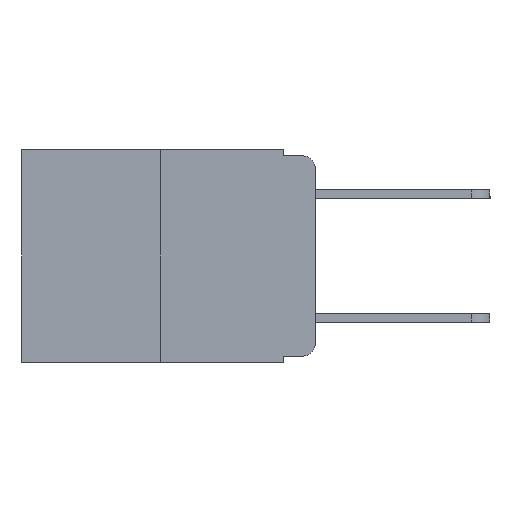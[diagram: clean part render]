
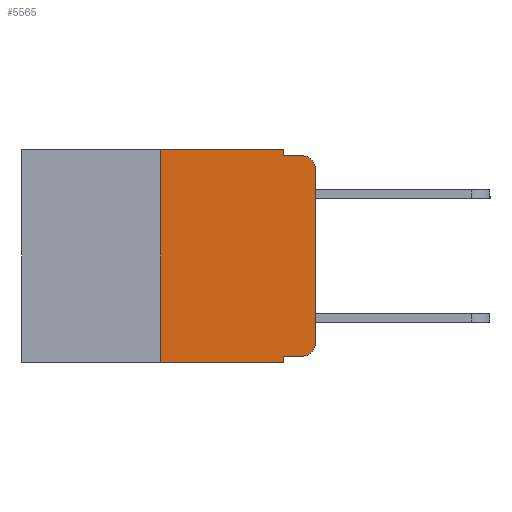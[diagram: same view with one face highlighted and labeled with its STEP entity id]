
A CAD part, left-side view. The second image highlights one B-rep face of the part: STEP entity #5565.
In plain terms, the highlighted planar face has unit normal (-1, 0, 0).
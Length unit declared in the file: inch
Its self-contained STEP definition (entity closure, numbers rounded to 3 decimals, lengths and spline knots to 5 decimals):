
#407 = EDGE_LOOP ( 'NONE', ( #6539, #4315, #10056, #1972, #2257, #2528, #5865, #9950, #4800, #1555 ) ) ;
#573 = EDGE_CURVE ( 'NONE', #8591, #6656, #7111, .T. ) ;
#878 = CARTESIAN_POINT ( 'NONE',  ( 0., 0.051, -0.333 ) ) ;
#940 = DIRECTION ( 'NONE',  ( 0., -1., 0. ) ) ;
#966 = CARTESIAN_POINT ( 'NONE',  ( 0., 0.051, -0.01 ) ) ;
#1211 = LINE ( 'NONE', #8106, #3371 ) ;
#1301 = CARTESIAN_POINT ( 'NONE',  ( 0., 0.051, -0.343 ) ) ;
#1351 = CARTESIAN_POINT ( 'NONE',  ( 0., 0.02, -0.01 ) ) ;
#1364 = VECTOR ( 'NONE', #940, 39.37008 ) ;
#1408 = VERTEX_POINT ( 'NONE', #9656 ) ;
#1488 = LINE ( 'NONE', #966, #3985 ) ;
#1555 = ORIENTED_EDGE ( 'NONE', *, *, #7581, .T. ) ;
#1786 = VECTOR ( 'NONE', #3696, 39.37008 ) ;
#1876 = CARTESIAN_POINT ( 'NONE',  ( 0., 0.473, -0.343 ) ) ;
#1972 = ORIENTED_EDGE ( 'NONE', *, *, #8365, .F. ) ;
#2257 = ORIENTED_EDGE ( 'NONE', *, *, #573, .F. ) ;
#2528 = ORIENTED_EDGE ( 'NONE', *, *, #7565, .F. ) ;
#2631 = CARTESIAN_POINT ( 'NONE',  ( 0., 0., -0.03 ) ) ;
#2979 = CARTESIAN_POINT ( 'NONE',  ( 0., 0.051, 0. ) ) ;
#3092 = CIRCLE ( 'NONE', #4493, 0.02 ) ;
#3120 = VERTEX_POINT ( 'NONE', #8500 ) ;
#3288 = CARTESIAN_POINT ( 'NONE',  ( 0., 0.473, 0. ) ) ;
#3371 = VECTOR ( 'NONE', #8825, 39.37008 ) ;
#3408 = LINE ( 'NONE', #2979, #9492 ) ;
#3435 = VERTEX_POINT ( 'NONE', #1301 ) ;
#3675 = LINE ( 'NONE', #10227, #8004 ) ;
#3689 = VERTEX_POINT ( 'NONE', #2631 ) ;
#3696 = DIRECTION ( 'NONE',  ( 0., -1., 0. ) ) ;
#3859 = CARTESIAN_POINT ( 'NONE',  ( 0., 0.02, -0.313 ) ) ;
#3972 = DIRECTION ( 'NONE',  ( 0., 0., -1. ) ) ;
#3985 = VECTOR ( 'NONE', #7278, 39.37008 ) ;
#4072 = CARTESIAN_POINT ( 'NONE',  ( 0., 0.02, -0.03 ) ) ;
#4111 = CIRCLE ( 'NONE', #9367, 0.02 ) ;
#4242 = CARTESIAN_POINT ( 'NONE',  ( 0., 0.051, -0.333 ) ) ;
#4311 = FACE_OUTER_BOUND ( 'NONE', #407, .T. ) ;
#4315 = ORIENTED_EDGE ( 'NONE', *, *, #7671, .T. ) ;
#4463 = CARTESIAN_POINT ( 'NONE',  ( 0., 0., -0.313 ) ) ;
#4493 = AXIS2_PLACEMENT_3D ( 'NONE', #3859, #9572, #4832 ) ;
#4800 = ORIENTED_EDGE ( 'NONE', *, *, #7518, .T. ) ;
#4832 = DIRECTION ( 'NONE',  ( 0., 0., -1. ) ) ;
#5009 = DIRECTION ( 'NONE',  ( 0., 0., -1. ) ) ;
#5565 = ADVANCED_FACE ( 'NONE', ( #4311 ), #7453, .F. ) ;
#5682 = LINE ( 'NONE', #1876, #1364 ) ;
#5763 = DIRECTION ( 'NONE',  ( 0., 0., -1. ) ) ;
#5865 = ORIENTED_EDGE ( 'NONE', *, *, #6898, .T. ) ;
#5964 = VERTEX_POINT ( 'NONE', #6295 ) ;
#6295 = CARTESIAN_POINT ( 'NONE',  ( 0., 0.02, -0.333 ) ) ;
#6539 = ORIENTED_EDGE ( 'NONE', *, *, #7569, .T. ) ;
#6655 = CARTESIAN_POINT ( 'NONE',  ( 0., 0.051, 0. ) ) ;
#6656 = VERTEX_POINT ( 'NONE', #10417 ) ;
#6764 = VERTEX_POINT ( 'NONE', #4463 ) ;
#6855 = VECTOR ( 'NONE', #9995, 39.37008 ) ;
#6870 = LINE ( 'NONE', #878, #1786 ) ;
#6898 = EDGE_CURVE ( 'NONE', #1408, #3435, #5682, .T. ) ;
#7111 = LINE ( 'NONE', #8272, #6855 ) ;
#7202 = VERTEX_POINT ( 'NONE', #1351 ) ;
#7270 = VERTEX_POINT ( 'NONE', #4242 ) ;
#7278 = DIRECTION ( 'NONE',  ( 0., -1., 0. ) ) ;
#7453 = PLANE ( 'NONE',  #10186 ) ;
#7518 = EDGE_CURVE ( 'NONE', #7270, #5964, #6870, .T. ) ;
#7549 = EDGE_CURVE ( 'NONE', #3120, #7202, #1488, .T. ) ;
#7565 = EDGE_CURVE ( 'NONE', #1408, #8591, #3675, .T. ) ;
#7569 = EDGE_CURVE ( 'NONE', #6764, #3689, #1211, .T. ) ;
#7581 = EDGE_CURVE ( 'NONE', #5964, #6764, #3092, .T. ) ;
#7671 = EDGE_CURVE ( 'NONE', #3689, #7202, #4111, .T. ) ;
#8004 = VECTOR ( 'NONE', #10888, 39.37008 ) ;
#8106 = CARTESIAN_POINT ( 'NONE',  ( 0., 0., 0. ) ) ;
#8272 = CARTESIAN_POINT ( 'NONE',  ( 0., 0.473, 0. ) ) ;
#8365 = EDGE_CURVE ( 'NONE', #6656, #3120, #3408, .T. ) ;
#8500 = CARTESIAN_POINT ( 'NONE',  ( 0., 0.051, -0.01 ) ) ;
#8591 = VERTEX_POINT ( 'NONE', #10453 ) ;
#8786 = VECTOR ( 'NONE', #3972, 39.37008 ) ;
#8825 = DIRECTION ( 'NONE',  ( 0., 0., 1. ) ) ;
#9014 = LINE ( 'NONE', #6655, #8786 ) ;
#9209 = DIRECTION ( 'NONE',  ( 1., 0., 0. ) ) ;
#9367 = AXIS2_PLACEMENT_3D ( 'NONE', #4072, #9734, #5009 ) ;
#9460 = DIRECTION ( 'NONE',  ( 0., 0., -1. ) ) ;
#9492 = VECTOR ( 'NONE', #5763, 39.37008 ) ;
#9572 = DIRECTION ( 'NONE',  ( -1., 0., 0. ) ) ;
#9582 = EDGE_CURVE ( 'NONE', #7270, #3435, #9014, .T. ) ;
#9656 = CARTESIAN_POINT ( 'NONE',  ( 0., 0.25, -0.343 ) ) ;
#9734 = DIRECTION ( 'NONE',  ( -1., 0., 0. ) ) ;
#9950 = ORIENTED_EDGE ( 'NONE', *, *, #9582, .F. ) ;
#9995 = DIRECTION ( 'NONE',  ( 0., -1., 0. ) ) ;
#10056 = ORIENTED_EDGE ( 'NONE', *, *, #7549, .F. ) ;
#10186 = AXIS2_PLACEMENT_3D ( 'NONE', #3288, #9209, #9460 ) ;
#10227 = CARTESIAN_POINT ( 'NONE',  ( 0., 0.25, 0. ) ) ;
#10417 = CARTESIAN_POINT ( 'NONE',  ( 0., 0.051, 0. ) ) ;
#10453 = CARTESIAN_POINT ( 'NONE',  ( 0., 0.25, 0. ) ) ;
#10888 = DIRECTION ( 'NONE',  ( 0., 0., 1. ) ) ;
